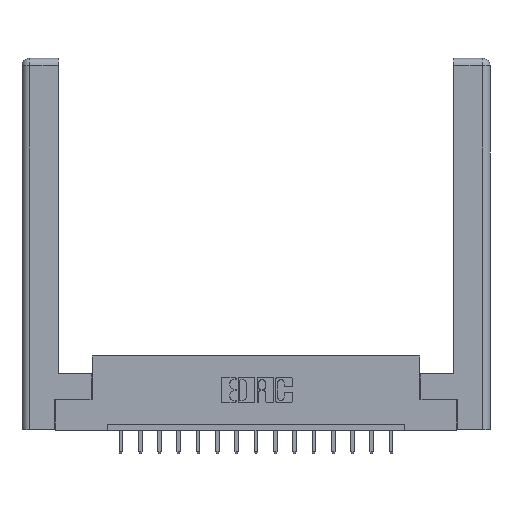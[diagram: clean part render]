
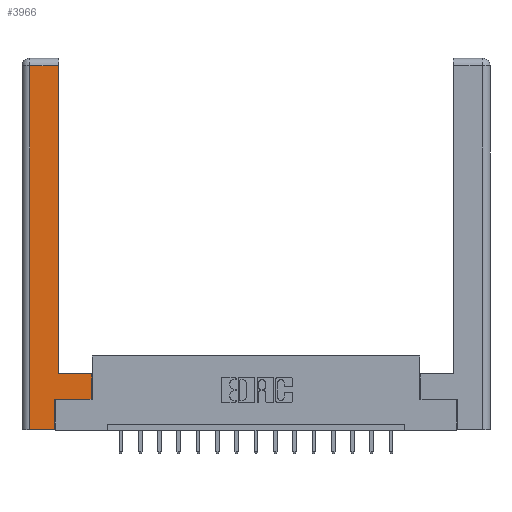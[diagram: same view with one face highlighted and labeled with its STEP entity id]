
A CAD part, top view. The second image highlights one B-rep face of the part: STEP entity #3966.
In plain terms, the highlighted planar face has unit normal (0, 0, 1).
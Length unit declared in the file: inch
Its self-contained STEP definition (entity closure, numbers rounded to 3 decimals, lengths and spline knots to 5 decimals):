
#108 = DIRECTION ( 'NONE',  ( 1., 0., 0. ) ) ;
#547 = VECTOR ( 'NONE', #4871, 39.37008 ) ;
#785 = VERTEX_POINT ( 'NONE', #17322 ) ;
#1046 = ORIENTED_EDGE ( 'NONE', *, *, #8728, .T. ) ;
#1096 = EDGE_CURVE ( 'NONE', #2545, #10711, #7755, .T. ) ;
#1448 = CARTESIAN_POINT ( 'NONE',  ( 0., 0., 0. ) ) ;
#1734 = LINE ( 'NONE', #2305, #10789 ) ;
#2305 = CARTESIAN_POINT ( 'NONE',  ( 0.295, 0.45, 0. ) ) ;
#2545 = VERTEX_POINT ( 'NONE', #12254 ) ;
#2715 = LINE ( 'NONE', #5680, #13450 ) ;
#3507 = VECTOR ( 'NONE', #5728, 39.37008 ) ;
#3966 = ADVANCED_FACE ( 'NONE', ( #16380 ), #8166, .F. ) ;
#4086 = DIRECTION ( 'NONE',  ( -1., 0., 0. ) ) ;
#4121 = CARTESIAN_POINT ( 'NONE',  ( 0.265, 0.245, 0. ) ) ;
#4725 = EDGE_CURVE ( 'NONE', #5988, #10616, #16130, .T. ) ;
#4871 = DIRECTION ( 'NONE',  ( 1., 0., 0. ) ) ;
#4970 = LINE ( 'NONE', #5553, #3507 ) ;
#5514 = CARTESIAN_POINT ( 'NONE',  ( 0.0615, 2.94, 0. ) ) ;
#5553 = CARTESIAN_POINT ( 'NONE',  ( 0.265, 0.245, 0. ) ) ;
#5612 = VECTOR ( 'NONE', #108, 39.37008 ) ;
#5680 = CARTESIAN_POINT ( 'NONE',  ( 0.565, 0.45, 0. ) ) ;
#5728 = DIRECTION ( 'NONE',  ( 0., 1., 0. ) ) ;
#5988 = VERTEX_POINT ( 'NONE', #4121 ) ;
#6538 = ORIENTED_EDGE ( 'NONE', *, *, #7054, .T. ) ;
#6639 = CARTESIAN_POINT ( 'NONE',  ( 0.295, 3., 0. ) ) ;
#6842 = DIRECTION ( 'NONE',  ( 0., 1., 0. ) ) ;
#6932 = CARTESIAN_POINT ( 'NONE',  ( 0.295, 0.45, 0. ) ) ;
#7054 = EDGE_CURVE ( 'NONE', #14761, #2545, #7220, .T. ) ;
#7220 = LINE ( 'NONE', #6639, #15826 ) ;
#7224 = CARTESIAN_POINT ( 'NONE',  ( 0.565, 0.245, 0. ) ) ;
#7482 = ORIENTED_EDGE ( 'NONE', *, *, #11369, .T. ) ;
#7755 = LINE ( 'NONE', #12312, #16782 ) ;
#8166 = PLANE ( 'NONE',  #10868 ) ;
#8409 = CARTESIAN_POINT ( 'NONE',  ( 0.0615, 0., 0. ) ) ;
#8728 = EDGE_CURVE ( 'NONE', #785, #5988, #4970, .T. ) ;
#9342 = DIRECTION ( 'NONE',  ( 0., 1., 0. ) ) ;
#9652 = LINE ( 'NONE', #16100, #5612 ) ;
#9711 = DIRECTION ( 'NONE',  ( 0., -1., 0. ) ) ;
#9759 = VERTEX_POINT ( 'NONE', #14004 ) ;
#9803 = ORIENTED_EDGE ( 'NONE', *, *, #4725, .T. ) ;
#10616 = VERTEX_POINT ( 'NONE', #7224 ) ;
#10703 = ORIENTED_EDGE ( 'NONE', *, *, #17178, .T. ) ;
#10711 = VERTEX_POINT ( 'NONE', #5514 ) ;
#10789 = VECTOR ( 'NONE', #14238, 39.37008 ) ;
#10857 = DIRECTION ( 'NONE',  ( -1., 0., 0. ) ) ;
#10868 = AXIS2_PLACEMENT_3D ( 'NONE', #1448, #13554, #10857 ) ;
#11222 = EDGE_LOOP ( 'NONE', ( #6538, #15425, #12445, #16651, #1046, #9803, #10703, #7482 ) ) ;
#11369 = EDGE_CURVE ( 'NONE', #9759, #14761, #1734, .T. ) ;
#12254 = CARTESIAN_POINT ( 'NONE',  ( 0.295, 2.94, 0. ) ) ;
#12312 = CARTESIAN_POINT ( 'NONE',  ( 0.0615, 2.94, 0. ) ) ;
#12445 = ORIENTED_EDGE ( 'NONE', *, *, #15835, .T. ) ;
#12446 = LINE ( 'NONE', #8409, #15573 ) ;
#12900 = CARTESIAN_POINT ( 'NONE',  ( 0.0615, 0., 0. ) ) ;
#13450 = VECTOR ( 'NONE', #6842, 39.37008 ) ;
#13474 = VERTEX_POINT ( 'NONE', #12900 ) ;
#13554 = DIRECTION ( 'NONE',  ( 0., 0., -1. ) ) ;
#14004 = CARTESIAN_POINT ( 'NONE',  ( 0.565, 0.45, 0. ) ) ;
#14181 = EDGE_CURVE ( 'NONE', #13474, #785, #9652, .T. ) ;
#14238 = DIRECTION ( 'NONE',  ( -1., 0., 0. ) ) ;
#14305 = CARTESIAN_POINT ( 'NONE',  ( 0.565, 0.245, 0. ) ) ;
#14761 = VERTEX_POINT ( 'NONE', #6932 ) ;
#15425 = ORIENTED_EDGE ( 'NONE', *, *, #1096, .T. ) ;
#15573 = VECTOR ( 'NONE', #9711, 39.37008 ) ;
#15826 = VECTOR ( 'NONE', #9342, 39.37008 ) ;
#15835 = EDGE_CURVE ( 'NONE', #10711, #13474, #12446, .T. ) ;
#16100 = CARTESIAN_POINT ( 'NONE',  ( 0.265, 0., 0. ) ) ;
#16130 = LINE ( 'NONE', #14305, #547 ) ;
#16380 = FACE_OUTER_BOUND ( 'NONE', #11222, .T. ) ;
#16651 = ORIENTED_EDGE ( 'NONE', *, *, #14181, .T. ) ;
#16782 = VECTOR ( 'NONE', #4086, 39.37008 ) ;
#17178 = EDGE_CURVE ( 'NONE', #10616, #9759, #2715, .T. ) ;
#17322 = CARTESIAN_POINT ( 'NONE',  ( 0.265, 0., 0. ) ) ;
